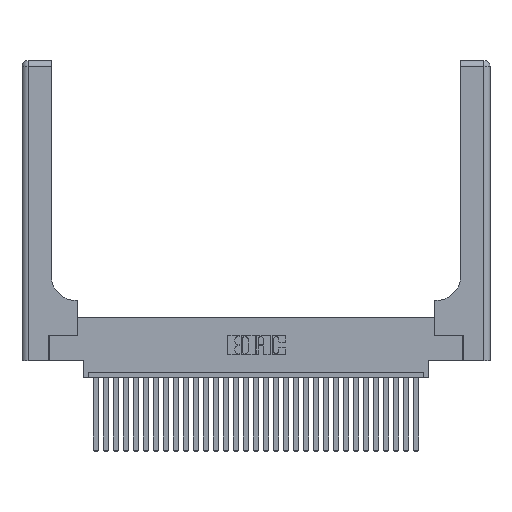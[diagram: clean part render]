
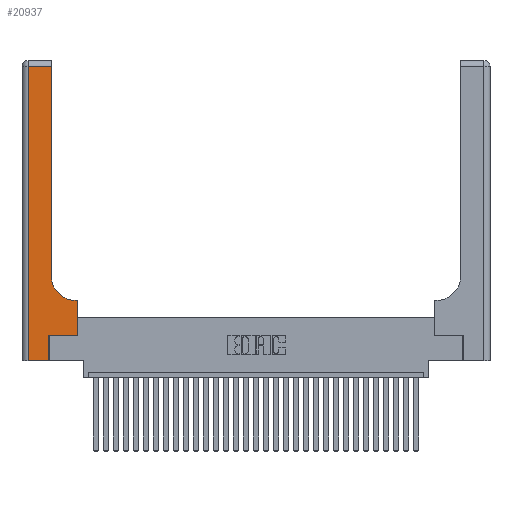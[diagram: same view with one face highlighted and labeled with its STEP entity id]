
A CAD part, top view. The second image highlights one B-rep face of the part: STEP entity #20937.
In plain terms, the highlighted planar face has unit normal (0, 0, 1).
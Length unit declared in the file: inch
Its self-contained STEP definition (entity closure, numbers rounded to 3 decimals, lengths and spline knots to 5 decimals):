
#166 = LINE ( 'NONE', #5973, #15299 ) ;
#252 = EDGE_CURVE ( 'NONE', #6149, #6572, #3423, .T. ) ;
#603 = VECTOR ( 'NONE', #13511, 39.37008 ) ;
#1470 = LINE ( 'NONE', #16478, #13553 ) ;
#1932 = VERTEX_POINT ( 'NONE', #25031 ) ;
#2051 = CARTESIAN_POINT ( 'NONE',  ( 0.5415, 0.85, 0.37 ) ) ;
#2576 = EDGE_CURVE ( 'NONE', #8528, #18453, #7075, .T. ) ;
#3150 = EDGE_CURVE ( 'NONE', #21457, #8528, #166, .T. ) ;
#3423 = LINE ( 'NONE', #3488, #29008 ) ;
#3488 = CARTESIAN_POINT ( 'NONE',  ( 0.2915, 3., 0.37 ) ) ;
#4517 = VERTEX_POINT ( 'NONE', #14450 ) ;
#4617 = DIRECTION ( 'NONE',  ( 0., 0., -1. ) ) ;
#5019 = CARTESIAN_POINT ( 'NONE',  ( 0.5585, 0.6, 0.37 ) ) ;
#5565 = EDGE_CURVE ( 'NONE', #6572, #19945, #1470, .T. ) ;
#5724 = CARTESIAN_POINT ( 'NONE',  ( 0.06, 0., 0.37 ) ) ;
#5868 = CARTESIAN_POINT ( 'NONE',  ( 0.06, 2.94, 0.37 ) ) ;
#5973 = CARTESIAN_POINT ( 'NONE',  ( 0.269, 0.25, 0.37 ) ) ;
#6149 = VERTEX_POINT ( 'NONE', #15973 ) ;
#6572 = VERTEX_POINT ( 'NONE', #19411 ) ;
#6589 = ORIENTED_EDGE ( 'NONE', *, *, #8562, .T. ) ;
#7075 = LINE ( 'NONE', #20998, #11945 ) ;
#7937 = ORIENTED_EDGE ( 'NONE', *, *, #252, .T. ) ;
#8041 = DIRECTION ( 'NONE',  ( 0., 1., 0. ) ) ;
#8528 = VERTEX_POINT ( 'NONE', #24536 ) ;
#8562 = EDGE_CURVE ( 'NONE', #4517, #6149, #19414, .T. ) ;
#8629 = PLANE ( 'NONE',  #25900 ) ;
#9333 = CARTESIAN_POINT ( 'NONE',  ( 0.2915, 0.6, 0.37 ) ) ;
#10955 = EDGE_CURVE ( 'NONE', #1932, #21457, #13992, .T. ) ;
#11784 = AXIS2_PLACEMENT_3D ( 'NONE', #2051, #4617, #14182 ) ;
#11945 = VECTOR ( 'NONE', #25714, 39.37008 ) ;
#13511 = DIRECTION ( 'NONE',  ( 0., -1., 0. ) ) ;
#13553 = VECTOR ( 'NONE', #21194, 39.37008 ) ;
#13992 = LINE ( 'NONE', #30940, #21915 ) ;
#14182 = DIRECTION ( 'NONE',  ( 1., 0., 0. ) ) ;
#14450 = CARTESIAN_POINT ( 'NONE',  ( 0.5415, 0.6, 0.37 ) ) ;
#14952 = LINE ( 'NONE', #23283, #603 ) ;
#15299 = VECTOR ( 'NONE', #25007, 39.37008 ) ;
#15328 = VERTEX_POINT ( 'NONE', #5724 ) ;
#15832 = EDGE_CURVE ( 'NONE', #15328, #1932, #25109, .T. ) ;
#15973 = CARTESIAN_POINT ( 'NONE',  ( 0.2915, 0.85, 0.37 ) ) ;
#16123 = VECTOR ( 'NONE', #21882, 39.37008 ) ;
#16478 = CARTESIAN_POINT ( 'NONE',  ( 0., 2.94, 0.37 ) ) ;
#17452 = CARTESIAN_POINT ( 'NONE',  ( 0., 0., 0.37 ) ) ;
#18453 = VERTEX_POINT ( 'NONE', #5019 ) ;
#18768 = ORIENTED_EDGE ( 'NONE', *, *, #5565, .T. ) ;
#19224 = LINE ( 'NONE', #9333, #28975 ) ;
#19411 = CARTESIAN_POINT ( 'NONE',  ( 0.2915, 2.94, 0.37 ) ) ;
#19414 = CIRCLE ( 'NONE', #11784, 0.25 ) ;
#19700 = DIRECTION ( 'NONE',  ( -1., 0., 0. ) ) ;
#19733 = EDGE_CURVE ( 'NONE', #19945, #15328, #14952, .T. ) ;
#19945 = VERTEX_POINT ( 'NONE', #5868 ) ;
#20937 = ADVANCED_FACE ( 'NONE', ( #31009 ), #8629, .F. ) ;
#20998 = CARTESIAN_POINT ( 'NONE',  ( 0.5585, 0.25, 0.37 ) ) ;
#21194 = DIRECTION ( 'NONE',  ( -1., 0., 0. ) ) ;
#21457 = VERTEX_POINT ( 'NONE', #22191 ) ;
#21882 = DIRECTION ( 'NONE',  ( 1., 0., 0. ) ) ;
#21915 = VECTOR ( 'NONE', #28102, 39.37008 ) ;
#22191 = CARTESIAN_POINT ( 'NONE',  ( 0.269, 0.25, 0.37 ) ) ;
#23283 = CARTESIAN_POINT ( 'NONE',  ( 0.06, 3., 0.37 ) ) ;
#23341 = EDGE_CURVE ( 'NONE', #18453, #4517, #19224, .T. ) ;
#24536 = CARTESIAN_POINT ( 'NONE',  ( 0.5585, 0.25, 0.37 ) ) ;
#25007 = DIRECTION ( 'NONE',  ( 1., 0., 0. ) ) ;
#25031 = CARTESIAN_POINT ( 'NONE',  ( 0.269, 0., 0.37 ) ) ;
#25109 = LINE ( 'NONE', #17452, #16123 ) ;
#25167 = ORIENTED_EDGE ( 'NONE', *, *, #2576, .T. ) ;
#25334 = DIRECTION ( 'NONE',  ( -1., 0., 0. ) ) ;
#25714 = DIRECTION ( 'NONE',  ( 0., 1., 0. ) ) ;
#25900 = AXIS2_PLACEMENT_3D ( 'NONE', #27941, #30253, #25334 ) ;
#26856 = EDGE_LOOP ( 'NONE', ( #7937, #18768, #28382, #27903, #30158, #30697, #25167, #27869, #6589 ) ) ;
#27869 = ORIENTED_EDGE ( 'NONE', *, *, #23341, .T. ) ;
#27903 = ORIENTED_EDGE ( 'NONE', *, *, #15832, .T. ) ;
#27941 = CARTESIAN_POINT ( 'NONE',  ( 0., 3., 0.37 ) ) ;
#28102 = DIRECTION ( 'NONE',  ( 0., 1., 0. ) ) ;
#28382 = ORIENTED_EDGE ( 'NONE', *, *, #19733, .T. ) ;
#28975 = VECTOR ( 'NONE', #19700, 39.37008 ) ;
#29008 = VECTOR ( 'NONE', #8041, 39.37008 ) ;
#30158 = ORIENTED_EDGE ( 'NONE', *, *, #10955, .T. ) ;
#30253 = DIRECTION ( 'NONE',  ( 0., 0., -1. ) ) ;
#30697 = ORIENTED_EDGE ( 'NONE', *, *, #3150, .T. ) ;
#30940 = CARTESIAN_POINT ( 'NONE',  ( 0.269, 0., 0.37 ) ) ;
#31009 = FACE_OUTER_BOUND ( 'NONE', #26856, .T. ) ;
